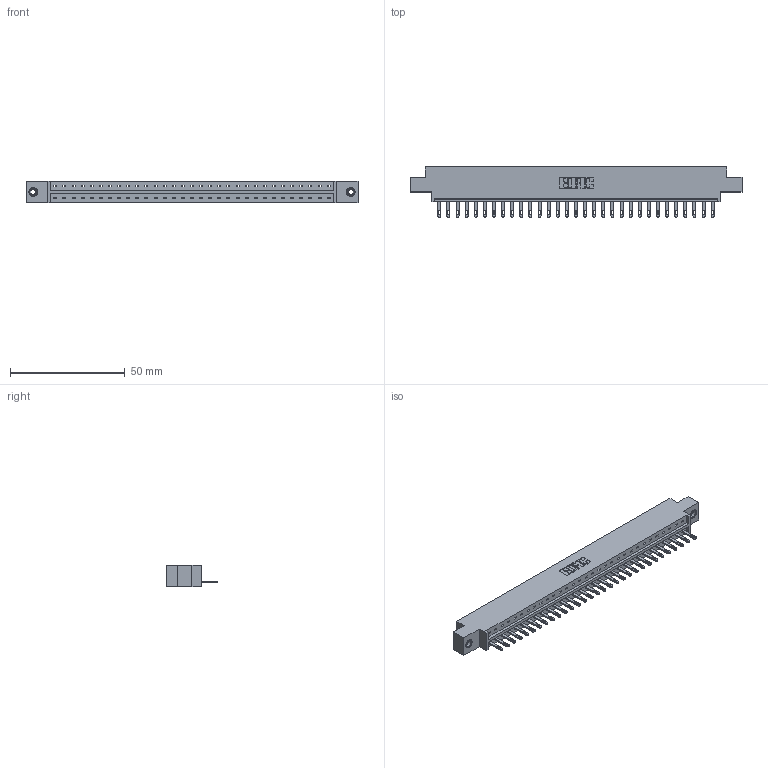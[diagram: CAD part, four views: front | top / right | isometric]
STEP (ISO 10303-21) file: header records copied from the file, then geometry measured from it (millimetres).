
FILE_DESCRIPTION (( 'STEP AP203' ), '1' );
FILE_NAME ('833-031-500-608.STEP', '2020-06-02T14:54:13', ( '' ), ( '' ), 'SwSTEP 2.0', 'SolidWorks 2020', '' );
FILE_SCHEMA (( 'CONFIG_CONTROL_DESIGN' ));
Length unit declared in the file: inch
Products named in the file (4): 833 Part_Offset - .156 Dia - TI; 345-250-001_345-250-003-102; 345-292-001_345-293-100; 833-031-500-608
Assembly tree (34 placements, depth 2):
  833-031-500-608
    833 Part_Offset - .156 Dia - TI
    345-292-001_345-293-100  x31
    345-250-001_345-250-003-102  x2
Bounding box: 144.37 x 21.85 x 9.4 mm (x, y, z)
Volume: 14218.3 mm3; surface area: 15611.1 mm2
Topology: 34 solids, 34 shells, 1852 faces, 5667 edges, 3770 vertices
Faces by surface type: plane 1222, cylinder 614, cone 12, torus 4
Entity records: 21622 total; most frequent: CARTESIAN_POINT 3714, ORIENTED_EDGE 3674, DIRECTION 3189, EDGE_CURVE 1837, VECTOR 1685, LINE 1685, VERTEX_POINT 1220, AXIS2_PLACEMENT_3D 752
